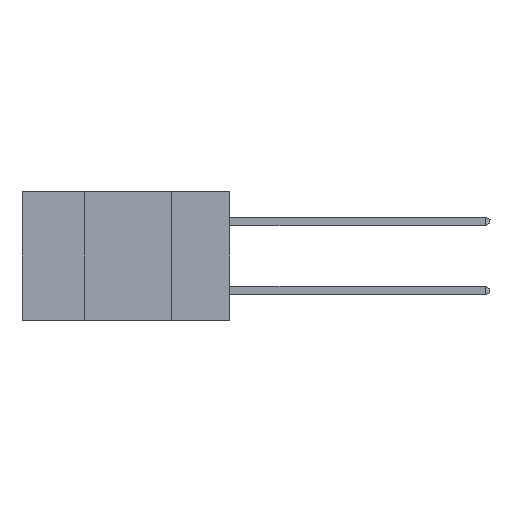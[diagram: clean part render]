
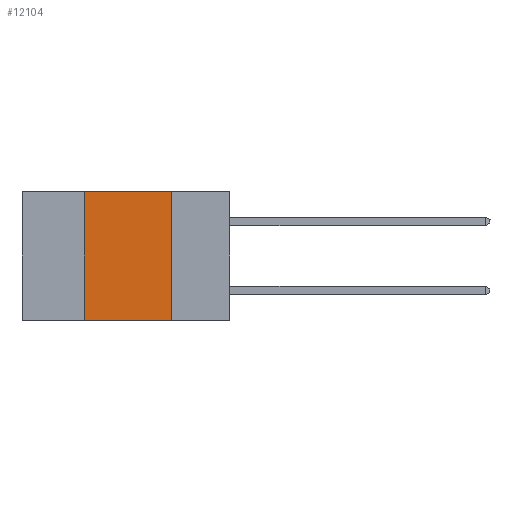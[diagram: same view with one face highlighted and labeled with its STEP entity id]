
A CAD part, left-side view. The second image highlights one B-rep face of the part: STEP entity #12104.
In plain terms, the highlighted planar face has unit normal (-1, 0, 0).
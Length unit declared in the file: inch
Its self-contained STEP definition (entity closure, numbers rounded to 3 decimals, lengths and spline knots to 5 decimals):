
#158 = DIRECTION ( 'NONE',  ( 0., -1., 0. ) ) ;
#323 = LINE ( 'NONE', #9891, #18702 ) ;
#655 = VECTOR ( 'NONE', #16455, 39.37008 ) ;
#700 = EDGE_CURVE ( 'NONE', #4564, #14108, #19402, .T. ) ;
#836 = PLANE ( 'NONE',  #2000 ) ;
#1644 = CARTESIAN_POINT ( 'NONE',  ( 0., 0.6, -0.37 ) ) ;
#1865 = CARTESIAN_POINT ( 'NONE',  ( 0., 0.42, -0.37 ) ) ;
#2000 = AXIS2_PLACEMENT_3D ( 'NONE', #18371, #7318, #15394 ) ;
#3071 = LINE ( 'NONE', #9556, #655 ) ;
#4472 = VERTEX_POINT ( 'NONE', #6717 ) ;
#4564 = VERTEX_POINT ( 'NONE', #15017 ) ;
#6717 = CARTESIAN_POINT ( 'NONE',  ( 0., 0.17, -0.37 ) ) ;
#7318 = DIRECTION ( 'NONE',  ( 1., 0., 0. ) ) ;
#8595 = EDGE_CURVE ( 'NONE', #4564, #4472, #19607, .T. ) ;
#8621 = EDGE_LOOP ( 'NONE', ( #9644, #12156, #15498, #12269 ) ) ;
#9556 = CARTESIAN_POINT ( 'NONE',  ( 0., 0.17, -0.37 ) ) ;
#9644 = ORIENTED_EDGE ( 'NONE', *, *, #12020, .F. ) ;
#9891 = CARTESIAN_POINT ( 'NONE',  ( 0., 0.6, 0. ) ) ;
#10292 = VECTOR ( 'NONE', #17901, 39.37008 ) ;
#12020 = EDGE_CURVE ( 'NONE', #16221, #4472, #3071, .T. ) ;
#12104 = ADVANCED_FACE ( 'NONE', ( #19969 ), #836, .F. ) ;
#12156 = ORIENTED_EDGE ( 'NONE', *, *, #16587, .F. ) ;
#12269 = ORIENTED_EDGE ( 'NONE', *, *, #8595, .T. ) ;
#14108 = VERTEX_POINT ( 'NONE', #16537 ) ;
#14781 = DIRECTION ( 'NONE',  ( 0., -1., 0. ) ) ;
#15017 = CARTESIAN_POINT ( 'NONE',  ( 0., 0.42, -0.37 ) ) ;
#15155 = CARTESIAN_POINT ( 'NONE',  ( 0., 0.17, 0. ) ) ;
#15394 = DIRECTION ( 'NONE',  ( 0., 0., -1. ) ) ;
#15498 = ORIENTED_EDGE ( 'NONE', *, *, #700, .F. ) ;
#16221 = VERTEX_POINT ( 'NONE', #15155 ) ;
#16455 = DIRECTION ( 'NONE',  ( 0., 0., -1. ) ) ;
#16537 = CARTESIAN_POINT ( 'NONE',  ( 0., 0.42, 0. ) ) ;
#16587 = EDGE_CURVE ( 'NONE', #14108, #16221, #323, .T. ) ;
#17610 = VECTOR ( 'NONE', #158, 39.37008 ) ;
#17901 = DIRECTION ( 'NONE',  ( 0., 0., 1. ) ) ;
#18371 = CARTESIAN_POINT ( 'NONE',  ( 0., 0.6, 0. ) ) ;
#18702 = VECTOR ( 'NONE', #14781, 39.37008 ) ;
#19402 = LINE ( 'NONE', #1865, #10292 ) ;
#19607 = LINE ( 'NONE', #1644, #17610 ) ;
#19969 = FACE_OUTER_BOUND ( 'NONE', #8621, .T. ) ;
